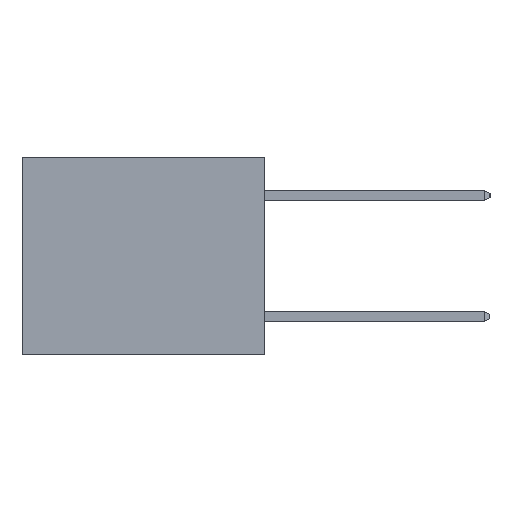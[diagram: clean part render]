
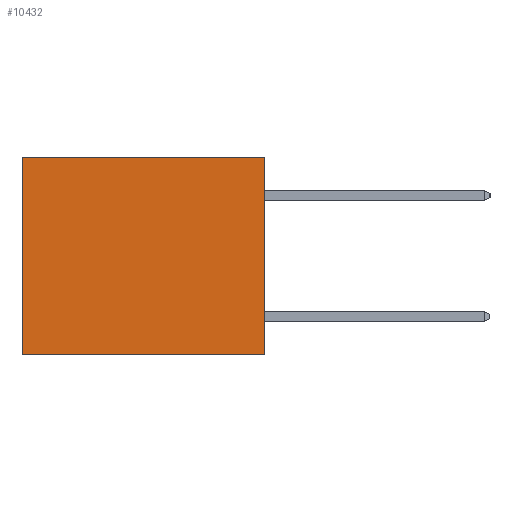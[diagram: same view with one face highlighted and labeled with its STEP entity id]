
A CAD part, left-side view. The second image highlights one B-rep face of the part: STEP entity #10432.
In plain terms, the highlighted planar face has unit normal (-1, 0, 0).
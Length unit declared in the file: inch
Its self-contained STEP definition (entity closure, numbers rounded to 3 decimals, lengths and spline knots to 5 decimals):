
#144 = CARTESIAN_POINT ( 'NONE',  ( 0.3165, 0., -0.49 ) ) ;
#374 = VERTEX_POINT ( 'NONE', #15006 ) ;
#548 = ORIENTED_EDGE ( 'NONE', *, *, #3280, .F. ) ;
#1334 = LINE ( 'NONE', #4522, #13028 ) ;
#1626 = EDGE_CURVE ( 'NONE', #9931, #374, #5762, .T. ) ;
#2738 = VERTEX_POINT ( 'NONE', #9936 ) ;
#3280 = EDGE_CURVE ( 'NONE', #9211, #2738, #13736, .T. ) ;
#4522 = CARTESIAN_POINT ( 'NONE',  ( 0.3165, 0., 0. ) ) ;
#5342 = CARTESIAN_POINT ( 'NONE',  ( 0.3165, 0., -0.49 ) ) ;
#5762 = LINE ( 'NONE', #15636, #12932 ) ;
#6575 = VECTOR ( 'NONE', #12284, 39.37008 ) ;
#6615 = DIRECTION ( 'NONE',  ( 0., 0., -1. ) ) ;
#7773 = VECTOR ( 'NONE', #13480, 39.37008 ) ;
#7778 = DIRECTION ( 'NONE',  ( 0., 0., -1. ) ) ;
#8235 = DIRECTION ( 'NONE',  ( 0., 1., 0. ) ) ;
#8370 = AXIS2_PLACEMENT_3D ( 'NONE', #5342, #12000, #6615 ) ;
#8447 = CARTESIAN_POINT ( 'NONE',  ( 0.3165, 0., 0. ) ) ;
#9211 = VERTEX_POINT ( 'NONE', #8447 ) ;
#9931 = VERTEX_POINT ( 'NONE', #11216 ) ;
#9936 = CARTESIAN_POINT ( 'NONE',  ( 0.3165, 0., -0.49 ) ) ;
#10272 = EDGE_LOOP ( 'NONE', ( #15211, #14890, #548, #15883 ) ) ;
#10432 = ADVANCED_FACE ( 'NONE', ( #12110 ), #11700, .F. ) ;
#10976 = CARTESIAN_POINT ( 'NONE',  ( 0.3165, 0., -0.49 ) ) ;
#11216 = CARTESIAN_POINT ( 'NONE',  ( 0.3165, 0.6, 0. ) ) ;
#11365 = EDGE_CURVE ( 'NONE', #2738, #374, #12923, .T. ) ;
#11700 = PLANE ( 'NONE',  #8370 ) ;
#12000 = DIRECTION ( 'NONE',  ( 1., 0., 0. ) ) ;
#12110 = FACE_OUTER_BOUND ( 'NONE', #10272, .T. ) ;
#12284 = DIRECTION ( 'NONE',  ( 0., 1., 0. ) ) ;
#12923 = LINE ( 'NONE', #10976, #6575 ) ;
#12932 = VECTOR ( 'NONE', #7778, 39.37008 ) ;
#13028 = VECTOR ( 'NONE', #8235, 39.37008 ) ;
#13480 = DIRECTION ( 'NONE',  ( 0., 0., -1. ) ) ;
#13736 = LINE ( 'NONE', #144, #7773 ) ;
#14757 = EDGE_CURVE ( 'NONE', #9211, #9931, #1334, .T. ) ;
#14890 = ORIENTED_EDGE ( 'NONE', *, *, #11365, .F. ) ;
#15006 = CARTESIAN_POINT ( 'NONE',  ( 0.3165, 0.6, -0.49 ) ) ;
#15211 = ORIENTED_EDGE ( 'NONE', *, *, #1626, .T. ) ;
#15636 = CARTESIAN_POINT ( 'NONE',  ( 0.3165, 0.6, -0.49 ) ) ;
#15883 = ORIENTED_EDGE ( 'NONE', *, *, #14757, .T. ) ;
